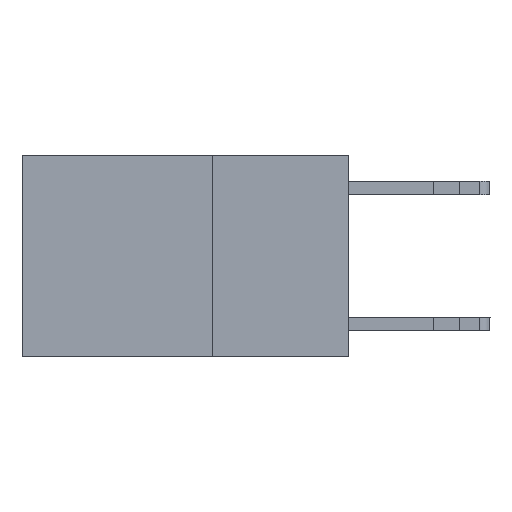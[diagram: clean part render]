
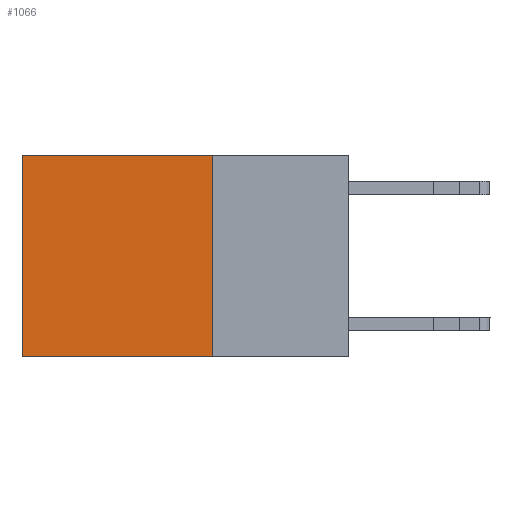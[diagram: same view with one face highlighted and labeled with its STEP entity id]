
A CAD part, left-side view. The second image highlights one B-rep face of the part: STEP entity #1066.
In plain terms, the highlighted planar face has unit normal (-1, 0, 0).
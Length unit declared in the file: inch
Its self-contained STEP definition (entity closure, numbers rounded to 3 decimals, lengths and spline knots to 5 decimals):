
#608 = VERTEX_POINT ( 'NONE', #10032 ) ;
#1066 = ADVANCED_FACE ( 'NONE', ( #4275 ), #1713, .F. ) ;
#1713 = PLANE ( 'NONE',  #4707 ) ;
#1816 = DIRECTION ( 'NONE',  ( 0., 0., -1. ) ) ;
#1841 = ORIENTED_EDGE ( 'NONE', *, *, #10730, .F. ) ;
#1957 = ORIENTED_EDGE ( 'NONE', *, *, #9836, .F. ) ;
#2031 = ORIENTED_EDGE ( 'NONE', *, *, #5278, .T. ) ;
#2046 = DIRECTION ( 'NONE',  ( 0., 1., 0. ) ) ;
#2749 = CARTESIAN_POINT ( 'NONE',  ( 0.2625, 0.25, 0. ) ) ;
#3083 = CARTESIAN_POINT ( 'NONE',  ( 0.2625, 0.25, 0. ) ) ;
#3306 = LINE ( 'NONE', #7945, #8412 ) ;
#3701 = DIRECTION ( 'NONE',  ( 0., 1., 0. ) ) ;
#3738 = VECTOR ( 'NONE', #3701, 39.37008 ) ;
#3748 = DIRECTION ( 'NONE',  ( 1., 0., 0. ) ) ;
#4275 = FACE_OUTER_BOUND ( 'NONE', #5913, .T. ) ;
#4707 = AXIS2_PLACEMENT_3D ( 'NONE', #2749, #3748, #10687 ) ;
#4782 = LINE ( 'NONE', #3083, #9818 ) ;
#5102 = VECTOR ( 'NONE', #10999, 39.37008 ) ;
#5278 = EDGE_CURVE ( 'NONE', #9041, #608, #4782, .T. ) ;
#5913 = EDGE_LOOP ( 'NONE', ( #12297, #1841, #1957, #2031 ) ) ;
#6527 = LINE ( 'NONE', #9744, #3738 ) ;
#7031 = VERTEX_POINT ( 'NONE', #9705 ) ;
#7433 = EDGE_CURVE ( 'NONE', #608, #9076, #12729, .T. ) ;
#7945 = CARTESIAN_POINT ( 'NONE',  ( 0.2625, 0.25, 0. ) ) ;
#8412 = VECTOR ( 'NONE', #1816, 39.37008 ) ;
#9041 = VERTEX_POINT ( 'NONE', #10874 ) ;
#9076 = VERTEX_POINT ( 'NONE', #11866 ) ;
#9705 = CARTESIAN_POINT ( 'NONE',  ( 0.2625, 0.25, -0.37 ) ) ;
#9744 = CARTESIAN_POINT ( 'NONE',  ( 0.2625, 0.25, -0.37 ) ) ;
#9818 = VECTOR ( 'NONE', #2046, 39.37008 ) ;
#9836 = EDGE_CURVE ( 'NONE', #9041, #7031, #3306, .T. ) ;
#10032 = CARTESIAN_POINT ( 'NONE',  ( 0.2625, 0.6, 0. ) ) ;
#10687 = DIRECTION ( 'NONE',  ( 0., 0., -1. ) ) ;
#10730 = EDGE_CURVE ( 'NONE', #7031, #9076, #6527, .T. ) ;
#10874 = CARTESIAN_POINT ( 'NONE',  ( 0.2625, 0.25, 0. ) ) ;
#10999 = DIRECTION ( 'NONE',  ( 0., 0., -1. ) ) ;
#11866 = CARTESIAN_POINT ( 'NONE',  ( 0.2625, 0.6, -0.37 ) ) ;
#11880 = CARTESIAN_POINT ( 'NONE',  ( 0.2625, 0.6, 0. ) ) ;
#12297 = ORIENTED_EDGE ( 'NONE', *, *, #7433, .T. ) ;
#12729 = LINE ( 'NONE', #11880, #5102 ) ;
